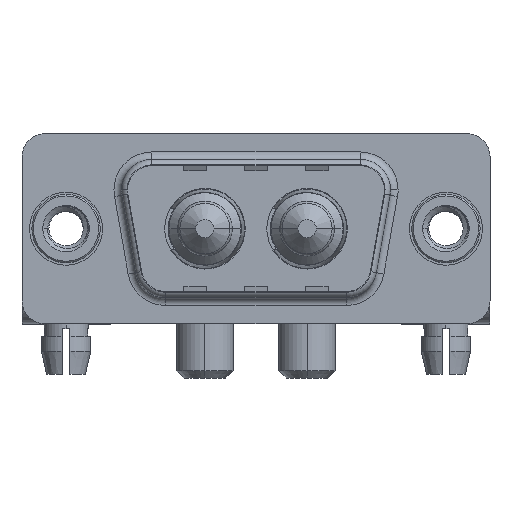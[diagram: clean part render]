
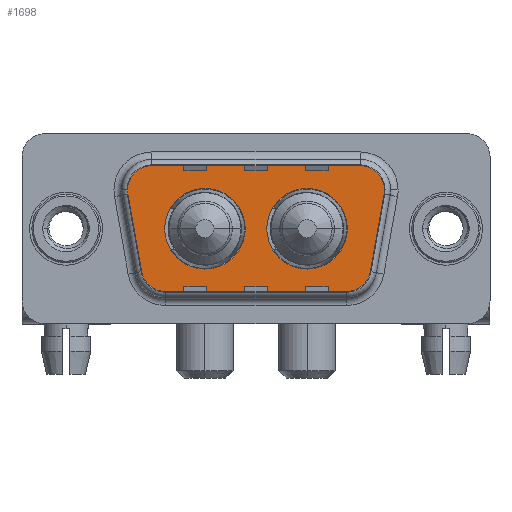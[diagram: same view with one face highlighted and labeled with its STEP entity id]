
A CAD part, top view. The second image highlights one B-rep face of the part: STEP entity #1698.
In plain terms, the highlighted planar face has unit normal (0, 0, 1).
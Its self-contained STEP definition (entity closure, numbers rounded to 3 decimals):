
#281 = CARTESIAN_POINT ( 'NONE',  ( 9.14, 0., 0. ) ) ;
#323 = DIRECTION ( 'NONE',  ( -1., 0., 0. ) ) ;
#350 = ORIENTED_EDGE ( 'NONE', *, *, #593, .F. ) ;
#375 = LINE ( 'NONE', #9831, #2138 ) ;
#425 = VERTEX_POINT ( 'NONE', #7432 ) ;
#559 = CIRCLE ( 'NONE', #7636, 2. ) ;
#593 = EDGE_CURVE ( 'NONE', #11108, #4843, #13464, .T. ) ;
#668 = DIRECTION ( 'NONE',  ( 0., 0., 1. ) ) ;
#780 = CIRCLE ( 'NONE', #4919, 2. ) ;
#855 = CARTESIAN_POINT ( 'NONE',  ( 11.79, 0., 0. ) ) ;
#856 = LINE ( 'NONE', #5514, #11824 ) ;
#1101 = DIRECTION ( 'NONE',  ( -1., 0., 0. ) ) ;
#1215 = CIRCLE ( 'NONE', #10717, 2. ) ;
#1259 = CARTESIAN_POINT ( 'NONE',  ( 20.511, -3.247, 0. ) ) ;
#1698 = ADVANCED_FACE ( 'NONE', ( #7810, #14606, #10023 ), #14759, .T. ) ;
#1709 = ORIENTED_EDGE ( 'NONE', *, *, #14000, .T. ) ;
#1729 = CIRCLE ( 'NONE', #4885, 2.65 ) ;
#1792 = CARTESIAN_POINT ( 'NONE',  ( 18.541, -2.9, 0. ) ) ;
#2020 = AXIS2_PLACEMENT_3D ( 'NONE', #9120, #14157, #12234 ) ;
#2138 = VECTOR ( 'NONE', #5025, 1000. ) ;
#2251 = CARTESIAN_POINT ( 'NONE',  ( 6.459, -2.9, 0. ) ) ;
#2596 = ORIENTED_EDGE ( 'NONE', *, *, #11828, .F. ) ;
#2667 = VERTEX_POINT ( 'NONE', #7639 ) ;
#2798 = EDGE_CURVE ( 'NONE', #8222, #425, #7998, .T. ) ;
#2856 = DIRECTION ( 'NONE',  ( 1., 0., 0. ) ) ;
#3005 = CIRCLE ( 'NONE', #2020, 2.65 ) ;
#3041 = VERTEX_POINT ( 'NONE', #14630 ) ;
#3485 = DIRECTION ( 'NONE',  ( 1., 0., 0. ) ) ;
#3506 = CARTESIAN_POINT ( 'NONE',  ( 5.436, 2.9, 0. ) ) ;
#3518 = VERTEX_POINT ( 'NONE', #855 ) ;
#3660 = CARTESIAN_POINT ( 'NONE',  ( 13.21, 0., 0. ) ) ;
#3736 = EDGE_LOOP ( 'NONE', ( #350, #14798 ) ) ;
#3957 = VECTOR ( 'NONE', #8062, 1000. ) ;
#4135 = VECTOR ( 'NONE', #7928, 1000. ) ;
#4174 = DIRECTION ( 'NONE',  ( -1., 0., 0. ) ) ;
#4316 = EDGE_CURVE ( 'NONE', #10038, #3041, #780, .T. ) ;
#4382 = DIRECTION ( 'NONE',  ( 0., 0., 1. ) ) ;
#4400 = VERTEX_POINT ( 'NONE', #8967 ) ;
#4627 = ORIENTED_EDGE ( 'NONE', *, *, #13627, .T. ) ;
#4666 = ORIENTED_EDGE ( 'NONE', *, *, #6446, .T. ) ;
#4834 = AXIS2_PLACEMENT_3D ( 'NONE', #7266, #10778, #323 ) ;
#4843 = VERTEX_POINT ( 'NONE', #3660 ) ;
#4877 = AXIS2_PLACEMENT_3D ( 'NONE', #14565, #668, #4174 ) ;
#4885 = AXIS2_PLACEMENT_3D ( 'NONE', #10019, #7438, #2856 ) ;
#4919 = AXIS2_PLACEMENT_3D ( 'NONE', #2251, #13786, #1101 ) ;
#5025 = DIRECTION ( 'NONE',  ( -1., 0., 0. ) ) ;
#5345 = ORIENTED_EDGE ( 'NONE', *, *, #6373, .T. ) ;
#5514 = CARTESIAN_POINT ( 'NONE',  ( 6.459, -4.9, 0. ) ) ;
#6049 = CIRCLE ( 'NONE', #11657, 2.65 ) ;
#6224 = VERTEX_POINT ( 'NONE', #12357 ) ;
#6373 = EDGE_CURVE ( 'NONE', #8535, #10038, #7071, .T. ) ;
#6446 = EDGE_CURVE ( 'NONE', #12500, #8222, #559, .T. ) ;
#6478 = ORIENTED_EDGE ( 'NONE', *, *, #6965, .F. ) ;
#6504 = CARTESIAN_POINT ( 'NONE',  ( 21.564, 2.9, 0. ) ) ;
#6724 = DIRECTION ( 'NONE',  ( 1., 0., 0. ) ) ;
#6805 = CARTESIAN_POINT ( 'NONE',  ( 3.466, 2.553, 0. ) ) ;
#6930 = CARTESIAN_POINT ( 'NONE',  ( 21.534, 2.553, 0. ) ) ;
#6965 = EDGE_CURVE ( 'NONE', #3518, #2667, #3005, .T. ) ;
#7071 = LINE ( 'NONE', #10583, #3957 ) ;
#7266 = CARTESIAN_POINT ( 'NONE',  ( 19.564, 2.9, 0. ) ) ;
#7293 = CARTESIAN_POINT ( 'NONE',  ( 18.541, -2.9, 0. ) ) ;
#7432 = CARTESIAN_POINT ( 'NONE',  ( 21.534, 2.553, 0. ) ) ;
#7438 = DIRECTION ( 'NONE',  ( 0., 0., 1. ) ) ;
#7511 = DIRECTION ( 'NONE',  ( 0., 0., 1. ) ) ;
#7537 = CARTESIAN_POINT ( 'NONE',  ( 4.489, -3.247, 0. ) ) ;
#7636 = AXIS2_PLACEMENT_3D ( 'NONE', #7293, #9512, #10808 ) ;
#7639 = CARTESIAN_POINT ( 'NONE',  ( 6.49, 0., 0. ) ) ;
#7794 = CARTESIAN_POINT ( 'NONE',  ( 18.541, -4.9, 0. ) ) ;
#7810 = FACE_BOUND ( 'NONE', #3736, .T. ) ;
#7928 = DIRECTION ( 'NONE',  ( 0.174, 0.985, 0. ) ) ;
#7998 = LINE ( 'NONE', #6930, #4135 ) ;
#8062 = DIRECTION ( 'NONE',  ( 0.174, -0.985, 0. ) ) ;
#8160 = DIRECTION ( 'NONE',  ( 1., 0., 0. ) ) ;
#8222 = VERTEX_POINT ( 'NONE', #1259 ) ;
#8535 = VERTEX_POINT ( 'NONE', #6805 ) ;
#8755 = ORIENTED_EDGE ( 'NONE', *, *, #12207, .T. ) ;
#8967 = CARTESIAN_POINT ( 'NONE',  ( 5.436, 4.9, 0. ) ) ;
#9120 = CARTESIAN_POINT ( 'NONE',  ( 9.14, 0., 0. ) ) ;
#9127 = EDGE_CURVE ( 'NONE', #3041, #12500, #856, .T. ) ;
#9512 = DIRECTION ( 'NONE',  ( 0., 0., 1. ) ) ;
#9713 = EDGE_LOOP ( 'NONE', ( #6478, #2596 ) ) ;
#9831 = CARTESIAN_POINT ( 'NONE',  ( 5.436, 4.9, 0. ) ) ;
#9875 = DIRECTION ( 'NONE',  ( 1., 0., 0. ) ) ;
#10019 = CARTESIAN_POINT ( 'NONE',  ( 15.86, 0., 0. ) ) ;
#10023 = FACE_OUTER_BOUND ( 'NONE', #14186, .T. ) ;
#10038 = VERTEX_POINT ( 'NONE', #7537 ) ;
#10215 = ORIENTED_EDGE ( 'NONE', *, *, #9127, .T. ) ;
#10583 = CARTESIAN_POINT ( 'NONE',  ( 3.466, 2.553, 0. ) ) ;
#10717 = AXIS2_PLACEMENT_3D ( 'NONE', #3506, #13885, #8160 ) ;
#10778 = DIRECTION ( 'NONE',  ( 0., 0., 1. ) ) ;
#10808 = DIRECTION ( 'NONE',  ( 1., 0., 0. ) ) ;
#11108 = VERTEX_POINT ( 'NONE', #11290 ) ;
#11290 = CARTESIAN_POINT ( 'NONE',  ( 18.51, 0., 0. ) ) ;
#11378 = EDGE_CURVE ( 'NONE', #6224, #4400, #375, .T. ) ;
#11401 = CARTESIAN_POINT ( 'NONE',  ( 15.86, 0., 0. ) ) ;
#11657 = AXIS2_PLACEMENT_3D ( 'NONE', #281, #12034, #11953 ) ;
#11824 = VECTOR ( 'NONE', #6724, 1000. ) ;
#11828 = EDGE_CURVE ( 'NONE', #2667, #3518, #6049, .T. ) ;
#11946 = ORIENTED_EDGE ( 'NONE', *, *, #11378, .T. ) ;
#11953 = DIRECTION ( 'NONE',  ( 1., 0., 0. ) ) ;
#12034 = DIRECTION ( 'NONE',  ( 0., 0., 1. ) ) ;
#12207 = EDGE_CURVE ( 'NONE', #12512, #6224, #14828, .T. ) ;
#12234 = DIRECTION ( 'NONE',  ( 1., 0., 0. ) ) ;
#12357 = CARTESIAN_POINT ( 'NONE',  ( 19.564, 4.9, 0. ) ) ;
#12500 = VERTEX_POINT ( 'NONE', #7794 ) ;
#12512 = VERTEX_POINT ( 'NONE', #6504 ) ;
#12922 = ORIENTED_EDGE ( 'NONE', *, *, #4316, .T. ) ;
#12978 = AXIS2_PLACEMENT_3D ( 'NONE', #11401, #4382, #3485 ) ;
#13464 = CIRCLE ( 'NONE', #12978, 2.65 ) ;
#13627 = EDGE_CURVE ( 'NONE', #4400, #8535, #1215, .T. ) ;
#13786 = DIRECTION ( 'NONE',  ( 0., 0., 1. ) ) ;
#13885 = DIRECTION ( 'NONE',  ( 0., 0., 1. ) ) ;
#14000 = EDGE_CURVE ( 'NONE', #425, #12512, #14632, .T. ) ;
#14157 = DIRECTION ( 'NONE',  ( 0., 0., 1. ) ) ;
#14186 = EDGE_LOOP ( 'NONE', ( #4666, #14547, #1709, #8755, #11946, #4627, #5345, #12922, #10215 ) ) ;
#14494 = AXIS2_PLACEMENT_3D ( 'NONE', #1792, #7511, #9875 ) ;
#14547 = ORIENTED_EDGE ( 'NONE', *, *, #2798, .T. ) ;
#14565 = CARTESIAN_POINT ( 'NONE',  ( 19.564, 2.9, 0. ) ) ;
#14606 = FACE_BOUND ( 'NONE', #9713, .T. ) ;
#14630 = CARTESIAN_POINT ( 'NONE',  ( 6.459, -4.9, 0. ) ) ;
#14632 = CIRCLE ( 'NONE', #4877, 2. ) ;
#14759 = PLANE ( 'NONE',  #14494 ) ;
#14798 = ORIENTED_EDGE ( 'NONE', *, *, #14897, .F. ) ;
#14828 = CIRCLE ( 'NONE', #4834, 2. ) ;
#14897 = EDGE_CURVE ( 'NONE', #4843, #11108, #1729, .T. ) ;
